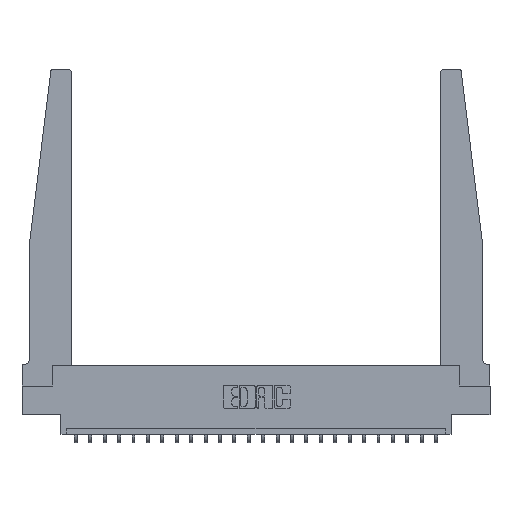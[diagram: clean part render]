
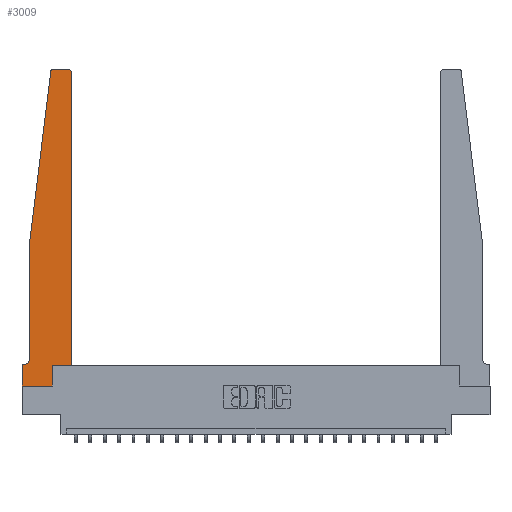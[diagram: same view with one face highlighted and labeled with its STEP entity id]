
A CAD part, top view. The second image highlights one B-rep face of the part: STEP entity #3009.
In plain terms, the highlighted planar face has unit normal (0, 0, 1).
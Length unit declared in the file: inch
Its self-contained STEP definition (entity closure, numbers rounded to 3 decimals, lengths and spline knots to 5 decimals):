
#68 = ORIENTED_EDGE ( 'NONE', *, *, #20530, .T. ) ;
#720 = DIRECTION ( 'NONE',  ( 1., 0., 0. ) ) ;
#907 = LINE ( 'NONE', #15524, #2668 ) ;
#1039 = DIRECTION ( 'NONE',  ( -1., 0., 0. ) ) ;
#1094 = DIRECTION ( 'NONE',  ( 0., 0., 1. ) ) ;
#1115 = DIRECTION ( 'NONE',  ( 1., 0., 0. ) ) ;
#1223 = CARTESIAN_POINT ( 'NONE',  ( 0.24675, 2.72367, 0.37 ) ) ;
#1243 = DIRECTION ( 'NONE',  ( 1., 0., 0. ) ) ;
#1372 = CARTESIAN_POINT ( 'NONE',  ( 0.425, 2.72, 0.37 ) ) ;
#1553 = VERTEX_POINT ( 'NONE', #18719 ) ;
#1801 = ORIENTED_EDGE ( 'NONE', *, *, #8467, .T. ) ;
#1959 = EDGE_CURVE ( 'NONE', #1553, #17978, #22305, .T. ) ;
#2582 = CARTESIAN_POINT ( 'NONE',  ( 0.425, 0.18, 0.37 ) ) ;
#2668 = VECTOR ( 'NONE', #22738, 39.37008 ) ;
#2953 = EDGE_CURVE ( 'NONE', #23072, #19470, #20944, .T. ) ;
#3009 = ADVANCED_FACE ( 'NONE', ( #9589 ), #16895, .T. ) ;
#3185 = CARTESIAN_POINT ( 'NONE',  ( 0.015, 0.2375, 0.37 ) ) ;
#3514 = CARTESIAN_POINT ( 'NONE',  ( 0.395, 2.72, 0.37 ) ) ;
#4954 = CIRCLE ( 'NONE', #17193, 0.03 ) ;
#5625 = AXIS2_PLACEMENT_3D ( 'NONE', #3514, #10829, #1243 ) ;
#5641 = CARTESIAN_POINT ( 'NONE',  ( 0.2605, 0.18, 0.37 ) ) ;
#5807 = ORIENTED_EDGE ( 'NONE', *, *, #6580, .T. ) ;
#5874 = DIRECTION ( 'NONE',  ( 1., 0., 0. ) ) ;
#5887 = CARTESIAN_POINT ( 'NONE',  ( 0., 0., 0.37 ) ) ;
#6109 = CARTESIAN_POINT ( 'NONE',  ( 0., 0.1875, 0.37 ) ) ;
#6580 = EDGE_CURVE ( 'NONE', #13545, #14833, #4954, .T. ) ;
#6676 = CARTESIAN_POINT ( 'NONE',  ( 0.015, 0.1875, 0.37 ) ) ;
#6946 = CARTESIAN_POINT ( 'NONE',  ( 0.065, 0.2375, 0.37 ) ) ;
#7324 = DIRECTION ( 'NONE',  ( -0.122, -0.992, 0. ) ) ;
#7797 = DIRECTION ( 'NONE',  ( 0., 0., 1. ) ) ;
#8261 = VECTOR ( 'NONE', #1115, 39.37008 ) ;
#8438 = CIRCLE ( 'NONE', #17631, 0.05 ) ;
#8446 = VECTOR ( 'NONE', #1039, 39.37008 ) ;
#8467 = EDGE_CURVE ( 'NONE', #20588, #19058, #19679, .T. ) ;
#8593 = CARTESIAN_POINT ( 'NONE',  ( 0.25, 2.75, 0.37 ) ) ;
#9125 = CARTESIAN_POINT ( 'NONE',  ( 0.065, 1.25, 0.37 ) ) ;
#9239 = VECTOR ( 'NONE', #7324, 39.37008 ) ;
#9589 = FACE_OUTER_BOUND ( 'NONE', #10769, .T. ) ;
#10160 = VECTOR ( 'NONE', #21863, 39.37008 ) ;
#10373 = DIRECTION ( 'NONE',  ( 0., 0., -1. ) ) ;
#10394 = ORIENTED_EDGE ( 'NONE', *, *, #2953, .T. ) ;
#10445 = DIRECTION ( 'NONE',  ( 1., 0., 0. ) ) ;
#10530 = CARTESIAN_POINT ( 'NONE',  ( 0.2605, 0.18, 0.37 ) ) ;
#10585 = CARTESIAN_POINT ( 'NONE',  ( 0.425, 0.18, 0.37 ) ) ;
#10769 = EDGE_LOOP ( 'NONE', ( #68, #5807, #21903, #13715, #16608, #1801, #19534, #22235, #21264, #21508, #21268, #10394 ) ) ;
#10829 = DIRECTION ( 'NONE',  ( 0., 0., 1. ) ) ;
#10856 = CARTESIAN_POINT ( 'NONE',  ( 0.395, 2.75, 0.37 ) ) ;
#10935 = EDGE_CURVE ( 'NONE', #21235, #11458, #907, .T. ) ;
#11458 = VERTEX_POINT ( 'NONE', #6946 ) ;
#12122 = CARTESIAN_POINT ( 'NONE',  ( 0.27653, 2.72, 0.37 ) ) ;
#12370 = LINE ( 'NONE', #9125, #9239 ) ;
#12483 = DIRECTION ( 'NONE',  ( -1., 0., 0. ) ) ;
#13335 = CARTESIAN_POINT ( 'NONE',  ( 0.065, 1.25, 0.37 ) ) ;
#13422 = EDGE_CURVE ( 'NONE', #11458, #20588, #8438, .T. ) ;
#13545 = VERTEX_POINT ( 'NONE', #14196 ) ;
#13715 = ORIENTED_EDGE ( 'NONE', *, *, #10935, .T. ) ;
#14196 = CARTESIAN_POINT ( 'NONE',  ( 0.27653, 2.75, 0.37 ) ) ;
#14237 = EDGE_CURVE ( 'NONE', #17978, #21686, #16025, .T. ) ;
#14752 = DIRECTION ( 'NONE',  ( 0., -1., 0. ) ) ;
#14833 = VERTEX_POINT ( 'NONE', #1223 ) ;
#15524 = CARTESIAN_POINT ( 'NONE',  ( 0.065, 1.25, 0.37 ) ) ;
#15766 = DIRECTION ( 'NONE',  ( -1., 0., 0. ) ) ;
#15799 = DIRECTION ( 'NONE',  ( 0., 1., 0. ) ) ;
#15809 = VERTEX_POINT ( 'NONE', #2582 ) ;
#15956 = CARTESIAN_POINT ( 'NONE',  ( 0.065, 0.1875, 0.37 ) ) ;
#16025 = LINE ( 'NONE', #10530, #16898 ) ;
#16608 = ORIENTED_EDGE ( 'NONE', *, *, #13422, .T. ) ;
#16668 = CARTESIAN_POINT ( 'NONE',  ( 0., 0., 0.37 ) ) ;
#16895 = PLANE ( 'NONE',  #22876 ) ;
#16898 = VECTOR ( 'NONE', #15799, 39.37008 ) ;
#17193 = AXIS2_PLACEMENT_3D ( 'NONE', #12122, #1094, #10445 ) ;
#17505 = CARTESIAN_POINT ( 'NONE',  ( 0.2605, 0., 0.37 ) ) ;
#17631 = AXIS2_PLACEMENT_3D ( 'NONE', #3185, #10373, #15766 ) ;
#17978 = VERTEX_POINT ( 'NONE', #17505 ) ;
#18588 = LINE ( 'NONE', #5887, #20400 ) ;
#18634 = VECTOR ( 'NONE', #5874, 39.37008 ) ;
#18719 = CARTESIAN_POINT ( 'NONE',  ( 0., 0., 0.37 ) ) ;
#18940 = EDGE_CURVE ( 'NONE', #21686, #15809, #21376, .T. ) ;
#19058 = VERTEX_POINT ( 'NONE', #22160 ) ;
#19470 = VERTEX_POINT ( 'NONE', #10856 ) ;
#19534 = ORIENTED_EDGE ( 'NONE', *, *, #22891, .T. ) ;
#19679 = LINE ( 'NONE', #15956, #22154 ) ;
#19734 = LINE ( 'NONE', #8593, #8446 ) ;
#19812 = LINE ( 'NONE', #21511, #10160 ) ;
#19863 = EDGE_CURVE ( 'NONE', #15809, #23072, #19812, .T. ) ;
#20400 = VECTOR ( 'NONE', #14752, 39.37008 ) ;
#20530 = EDGE_CURVE ( 'NONE', #19470, #13545, #19734, .T. ) ;
#20588 = VERTEX_POINT ( 'NONE', #6676 ) ;
#20944 = CIRCLE ( 'NONE', #5625, 0.03 ) ;
#21235 = VERTEX_POINT ( 'NONE', #13335 ) ;
#21264 = ORIENTED_EDGE ( 'NONE', *, *, #14237, .T. ) ;
#21268 = ORIENTED_EDGE ( 'NONE', *, *, #19863, .T. ) ;
#21376 = LINE ( 'NONE', #10585, #8261 ) ;
#21508 = ORIENTED_EDGE ( 'NONE', *, *, #18940, .T. ) ;
#21511 = CARTESIAN_POINT ( 'NONE',  ( 0.425, 0.18, 0.37 ) ) ;
#21686 = VERTEX_POINT ( 'NONE', #5641 ) ;
#21863 = DIRECTION ( 'NONE',  ( 0., 1., 0. ) ) ;
#21903 = ORIENTED_EDGE ( 'NONE', *, *, #22832, .T. ) ;
#22154 = VECTOR ( 'NONE', #12483, 39.37008 ) ;
#22160 = CARTESIAN_POINT ( 'NONE',  ( 0., 0.1875, 0.37 ) ) ;
#22235 = ORIENTED_EDGE ( 'NONE', *, *, #1959, .T. ) ;
#22305 = LINE ( 'NONE', #16668, #18634 ) ;
#22738 = DIRECTION ( 'NONE',  ( 0., -1., 0. ) ) ;
#22832 = EDGE_CURVE ( 'NONE', #14833, #21235, #12370, .T. ) ;
#22876 = AXIS2_PLACEMENT_3D ( 'NONE', #6109, #7797, #720 ) ;
#22891 = EDGE_CURVE ( 'NONE', #19058, #1553, #18588, .T. ) ;
#23072 = VERTEX_POINT ( 'NONE', #1372 ) ;
